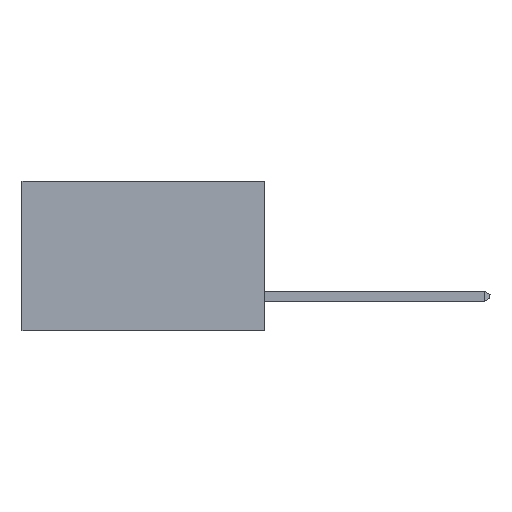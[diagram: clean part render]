
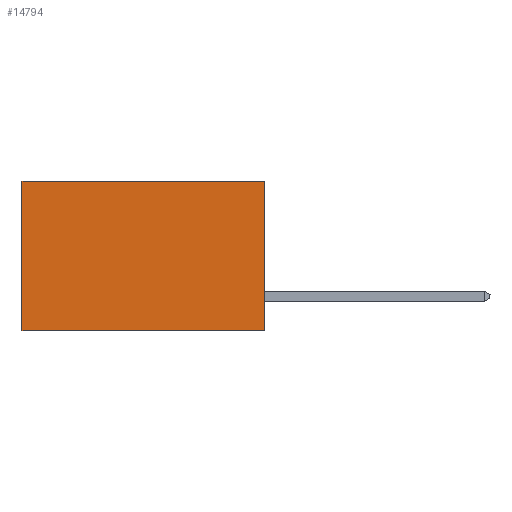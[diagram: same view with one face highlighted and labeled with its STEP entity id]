
A CAD part, left-side view. The second image highlights one B-rep face of the part: STEP entity #14794.
In plain terms, the highlighted planar face has unit normal (-1, 0, 0).
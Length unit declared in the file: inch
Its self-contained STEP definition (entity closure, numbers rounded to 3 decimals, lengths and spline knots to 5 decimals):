
#1119 = VERTEX_POINT ( 'NONE', #13958 ) ;
#2766 = VECTOR ( 'NONE', #16643, 39.37008 ) ;
#3131 = LINE ( 'NONE', #5116, #8611 ) ;
#3320 = AXIS2_PLACEMENT_3D ( 'NONE', #3589, #16552, #8797 ) ;
#3458 = CARTESIAN_POINT ( 'NONE',  ( 0.298, 0.6, -0.37 ) ) ;
#3539 = DIRECTION ( 'NONE',  ( 0., 0., -1. ) ) ;
#3589 = CARTESIAN_POINT ( 'NONE',  ( 0.298, 0., 0. ) ) ;
#4835 = PLANE ( 'NONE',  #3320 ) ;
#5116 = CARTESIAN_POINT ( 'NONE',  ( 0.298, 0., 0. ) ) ;
#5704 = EDGE_CURVE ( 'NONE', #1119, #14558, #10688, .T. ) ;
#6004 = EDGE_CURVE ( 'NONE', #15579, #14368, #14975, .T. ) ;
#6221 = CARTESIAN_POINT ( 'NONE',  ( 0.298, 0., -0.37 ) ) ;
#7163 = ORIENTED_EDGE ( 'NONE', *, *, #5704, .T. ) ;
#7955 = ORIENTED_EDGE ( 'NONE', *, *, #6004, .F. ) ;
#8382 = VECTOR ( 'NONE', #14043, 39.37008 ) ;
#8394 = ORIENTED_EDGE ( 'NONE', *, *, #13393, .F. ) ;
#8611 = VECTOR ( 'NONE', #14075, 39.37008 ) ;
#8797 = DIRECTION ( 'NONE',  ( 0., 0., -1. ) ) ;
#9261 = FACE_OUTER_BOUND ( 'NONE', #12702, .T. ) ;
#10688 = LINE ( 'NONE', #14046, #2766 ) ;
#12414 = ORIENTED_EDGE ( 'NONE', *, *, #15393, .T. ) ;
#12514 = VECTOR ( 'NONE', #3539, 39.37008 ) ;
#12702 = EDGE_LOOP ( 'NONE', ( #7163, #8394, #7955, #12414 ) ) ;
#13393 = EDGE_CURVE ( 'NONE', #14368, #14558, #15757, .T. ) ;
#13851 = CARTESIAN_POINT ( 'NONE',  ( 0.298, 0., 0. ) ) ;
#13958 = CARTESIAN_POINT ( 'NONE',  ( 0.298, 0.6, 0. ) ) ;
#14043 = DIRECTION ( 'NONE',  ( 0., 1., 0. ) ) ;
#14046 = CARTESIAN_POINT ( 'NONE',  ( 0.298, 0.6, 0. ) ) ;
#14075 = DIRECTION ( 'NONE',  ( 0., 1., 0. ) ) ;
#14368 = VERTEX_POINT ( 'NONE', #14934 ) ;
#14558 = VERTEX_POINT ( 'NONE', #3458 ) ;
#14794 = ADVANCED_FACE ( 'NONE', ( #9261 ), #4835, .F. ) ;
#14934 = CARTESIAN_POINT ( 'NONE',  ( 0.298, 0., -0.37 ) ) ;
#14975 = LINE ( 'NONE', #13851, #12514 ) ;
#15393 = EDGE_CURVE ( 'NONE', #15579, #1119, #3131, .T. ) ;
#15579 = VERTEX_POINT ( 'NONE', #15976 ) ;
#15757 = LINE ( 'NONE', #6221, #8382 ) ;
#15976 = CARTESIAN_POINT ( 'NONE',  ( 0.298, 0., 0. ) ) ;
#16552 = DIRECTION ( 'NONE',  ( 1., 0., 0. ) ) ;
#16643 = DIRECTION ( 'NONE',  ( 0., 0., -1. ) ) ;
